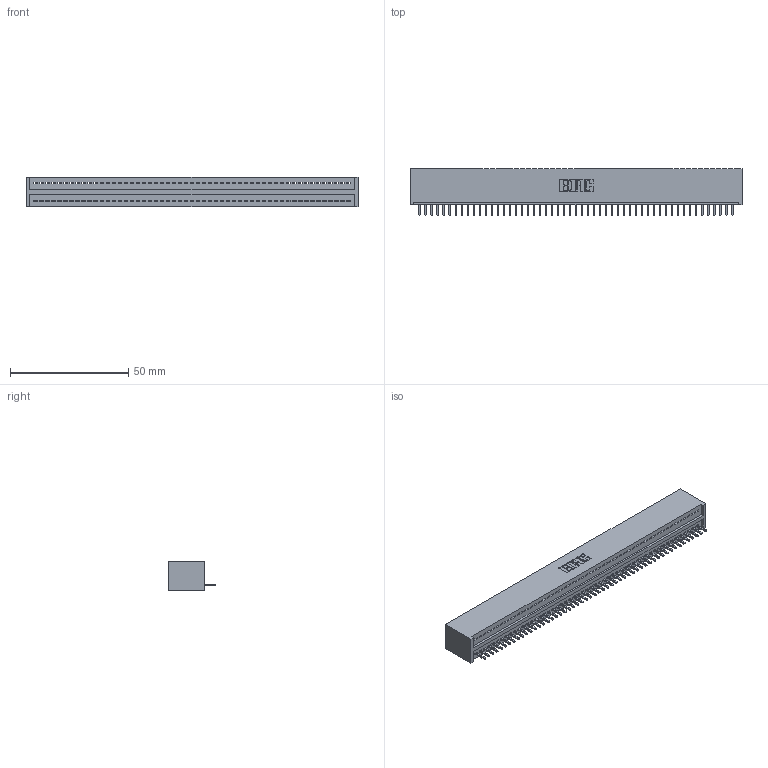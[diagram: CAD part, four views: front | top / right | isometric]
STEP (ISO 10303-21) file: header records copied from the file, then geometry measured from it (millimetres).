
FILE_DESCRIPTION (( 'STEP AP203' ), '1' );
FILE_NAME ('325-053-520-101.STEP', '2020-02-25T00:38:42', ( '' ), ( '' ), 'SwSTEP 2.0', 'SolidWorks 2016', '' );
FILE_SCHEMA (( 'CONFIG_CONTROL_DESIGN' ));
Length unit declared in the file: inch
Products named in the file (3): 325-053-520-101; 325-292-001_325-293-120; 325 Part_Lugless
Assembly tree (54 placements, depth 2):
  325-053-520-101
    325 Part_Lugless
    325-292-001_325-293-120  x53
Bounding box: 140.26 x 19.68 x 12.45 mm (x, y, z)
Volume: 18327.1 mm3; surface area: 20142 mm2
Topology: 54 solids, 54 shells, 3180 faces, 9615 edges, 6338 vertices
Faces by surface type: plane 2292, cylinder 888
Entity records: 30719 total; most frequent: CARTESIAN_POINT 5305, ORIENTED_EDGE 5294, DIRECTION 4445, EDGE_CURVE 2647, VECTOR 2527, LINE 2527, VERTEX_POINT 1762, AXIS2_PLACEMENT_3D 959
